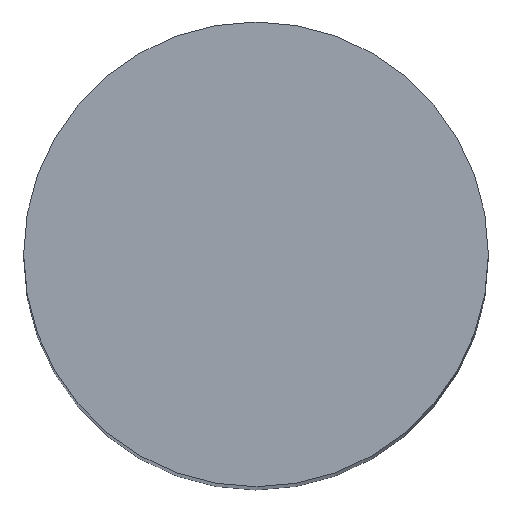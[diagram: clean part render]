
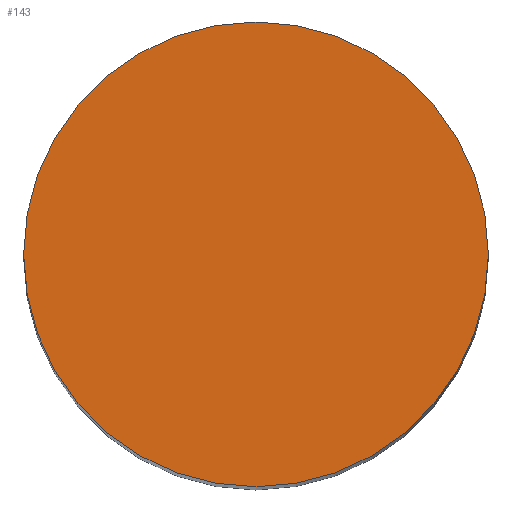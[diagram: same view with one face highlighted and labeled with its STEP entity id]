
A CAD part, top view. The second image highlights one B-rep face of the part: STEP entity #143.
In plain terms, the highlighted planar face has unit normal (0, 0, 1).
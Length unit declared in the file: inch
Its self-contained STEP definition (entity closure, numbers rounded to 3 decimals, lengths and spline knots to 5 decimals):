
#2 = AXIS2_PLACEMENT_3D ( 'NONE', #112, #108, #102 ) ;
#15 = EDGE_CURVE ( 'NONE', #34, #22, #135, .T. ) ;
#22 = VERTEX_POINT ( 'NONE', #128 ) ;
#28 = DIRECTION ( 'NONE',  ( 0., 0., 1. ) ) ;
#31 = DIRECTION ( 'NONE',  ( 1., 0., 0. ) ) ;
#34 = VERTEX_POINT ( 'NONE', #86 ) ;
#39 = PLANE ( 'NONE',  #56 ) ;
#43 = FACE_OUTER_BOUND ( 'NONE', #58, .T. ) ;
#44 = CARTESIAN_POINT ( 'NONE',  ( 0., 0., 6. ) ) ;
#56 = AXIS2_PLACEMENT_3D ( 'NONE', #44, #28, #31 ) ;
#58 = EDGE_LOOP ( 'NONE', ( #97, #100 ) ) ;
#64 = AXIS2_PLACEMENT_3D ( 'NONE', #105, #82, #69 ) ;
#67 = CIRCLE ( 'NONE', #2, 0.75 ) ;
#69 = DIRECTION ( 'NONE',  ( 1., 0., 0. ) ) ;
#82 = DIRECTION ( 'NONE',  ( 0., 0., 1. ) ) ;
#86 = CARTESIAN_POINT ( 'NONE',  ( 16.06546, 16.51113, 6. ) ) ;
#89 = EDGE_CURVE ( 'NONE', #22, #34, #67, .T. ) ;
#97 = ORIENTED_EDGE ( 'NONE', *, *, #15, .T. ) ;
#100 = ORIENTED_EDGE ( 'NONE', *, *, #89, .T. ) ;
#102 = DIRECTION ( 'NONE',  ( 1., 0., 0. ) ) ;
#105 = CARTESIAN_POINT ( 'NONE',  ( 16.81546, 16.51113, 6. ) ) ;
#108 = DIRECTION ( 'NONE',  ( 0., 0., 1. ) ) ;
#112 = CARTESIAN_POINT ( 'NONE',  ( 16.81546, 16.51113, 6. ) ) ;
#128 = CARTESIAN_POINT ( 'NONE',  ( 17.56546, 16.51113, 6. ) ) ;
#135 = CIRCLE ( 'NONE', #64, 0.75 ) ;
#143 = ADVANCED_FACE ( 'NONE', ( #43 ), #39, .T. ) ;
